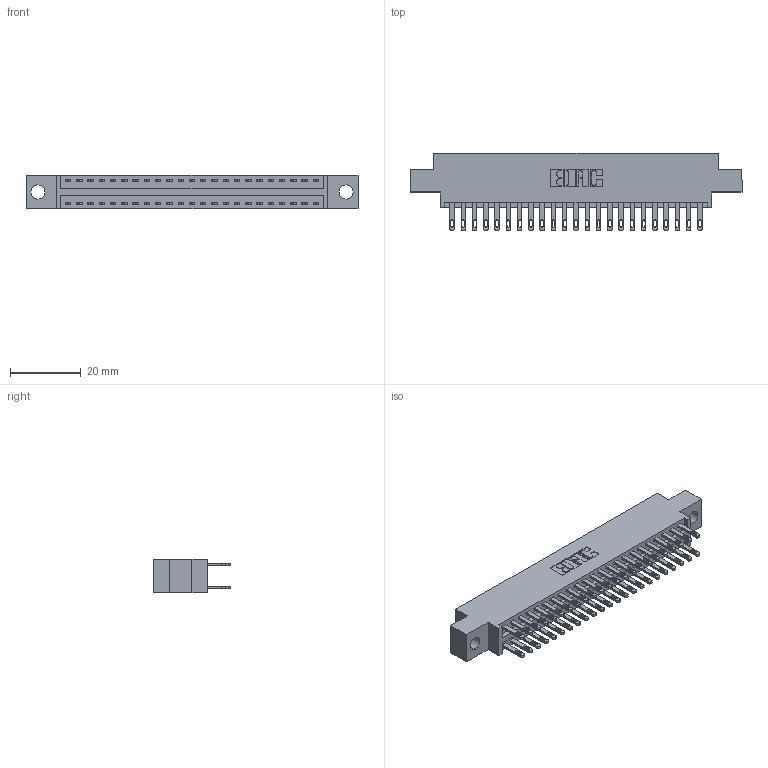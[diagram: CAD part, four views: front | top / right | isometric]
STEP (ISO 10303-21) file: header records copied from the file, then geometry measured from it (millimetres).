
FILE_DESCRIPTION (( 'STEP AP203' ), '1' );
FILE_NAME ('346-046-500-804.STEP', '2022-05-20T08:53:33', ( '' ), ( '' ), 'SwSTEP 2.0', 'SolidWorks 2020', '' );
FILE_SCHEMA (( 'CONFIG_CONTROL_DESIGN' ));
Length unit declared in the file: inch
Products named in the file (3): 346-046-500-804; 345-292-001_345-293-100; 346 Part_0.170 Offset - 0.156 Dia-TH
Assembly tree (47 placements, depth 2):
  346-046-500-804
    346 Part_0.170 Offset - 0.156 Dia-TH
    345-292-001_345-293-100  x46
Bounding box: 93.6 x 21.84 x 9.4 mm (x, y, z)
Volume: 8859.5 mm3; surface area: 12388.3 mm2
Topology: 47 solids, 47 shells, 2348 faces, 7139 edges, 4758 vertices
Faces by surface type: plane 1428, cylinder 920
Entity records: 18049 total; most frequent: CARTESIAN_POINT 3006, ORIENTED_EDGE 2938, DIRECTION 2701, EDGE_CURVE 1469, VECTOR 1241, LINE 1241, VERTEX_POINT 978, AXIS2_PLACEMENT_3D 730
